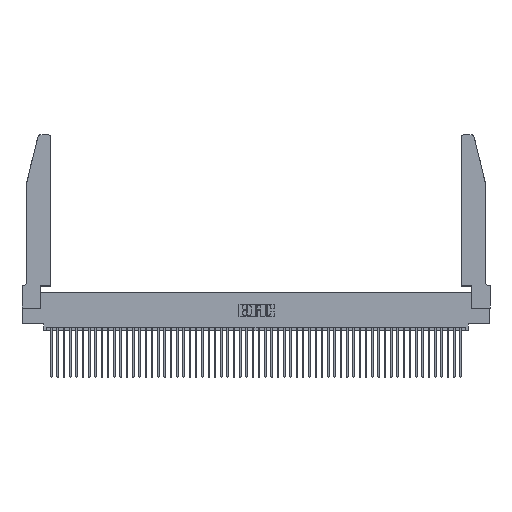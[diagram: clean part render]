
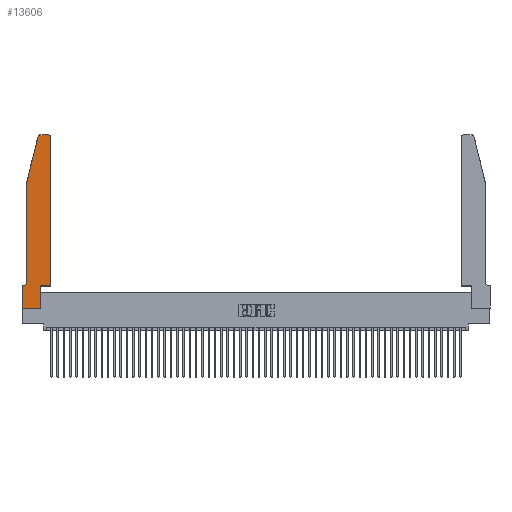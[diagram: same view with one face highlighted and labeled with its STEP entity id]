
A CAD part, top view. The second image highlights one B-rep face of the part: STEP entity #13606.
In plain terms, the highlighted planar face has unit normal (0, 0, 1).
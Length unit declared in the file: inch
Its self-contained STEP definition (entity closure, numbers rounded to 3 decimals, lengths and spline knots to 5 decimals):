
#648 = VERTEX_POINT ( 'NONE', #53403 ) ;
#2303 = EDGE_CURVE ( 'NONE', #8996, #44740, #25401, .T. ) ;
#3065 = ORIENTED_EDGE ( 'NONE', *, *, #2303, .T. ) ;
#3672 = CARTESIAN_POINT ( 'NONE',  ( 0.4505, 0.35, 0.37 ) ) ;
#4632 = AXIS2_PLACEMENT_3D ( 'NONE', #6742, #19001, #35114 ) ;
#5194 = CARTESIAN_POINT ( 'NONE',  ( 0.2865, 0., 0.37 ) ) ;
#5796 = LINE ( 'NONE', #16318, #37480 ) ;
#5951 = CARTESIAN_POINT ( 'NONE',  ( 0., 0., 0.37 ) ) ;
#6228 = CARTESIAN_POINT ( 'NONE',  ( 0.0055, 0.42, 0.37 ) ) ;
#6640 = AXIS2_PLACEMENT_3D ( 'NONE', #6228, #18672, #35143 ) ;
#6742 = CARTESIAN_POINT ( 'NONE',  ( 0.4205, 2.72, 0.37 ) ) ;
#7563 = EDGE_CURVE ( 'NONE', #29577, #43509, #40309, .T. ) ;
#8777 = VECTOR ( 'NONE', #47418, 39.37008 ) ;
#8996 = VERTEX_POINT ( 'NONE', #10641 ) ;
#9211 = DIRECTION ( 'NONE',  ( 0., 1., 0. ) ) ;
#9714 = DIRECTION ( 'NONE',  ( -0.239, -0.971, 0. ) ) ;
#9762 = EDGE_CURVE ( 'NONE', #44667, #41409, #36049, .T. ) ;
#10292 = LINE ( 'NONE', #13333, #30944 ) ;
#10329 = DIRECTION ( 'NONE',  ( -1., 0., 0. ) ) ;
#10641 = CARTESIAN_POINT ( 'NONE',  ( 0.25487, 2.72718, 0.37 ) ) ;
#10679 = EDGE_CURVE ( 'NONE', #43509, #648, #10292, .T. ) ;
#11545 = VERTEX_POINT ( 'NONE', #17422 ) ;
#12199 = ORIENTED_EDGE ( 'NONE', *, *, #41838, .T. ) ;
#12677 = CIRCLE ( 'NONE', #42104, 0.03 ) ;
#13333 = CARTESIAN_POINT ( 'NONE',  ( 0.2605, 2.75, 0.37 ) ) ;
#13467 = ORIENTED_EDGE ( 'NONE', *, *, #7563, .T. ) ;
#13606 = ADVANCED_FACE ( 'NONE', ( #36514 ), #26960, .T. ) ;
#13779 = CARTESIAN_POINT ( 'NONE',  ( 0.4505, 0.35, 0.37 ) ) ;
#13926 = CARTESIAN_POINT ( 'NONE',  ( 0.2865, 0.35, 0.37 ) ) ;
#13992 = VERTEX_POINT ( 'NONE', #14351 ) ;
#14351 = CARTESIAN_POINT ( 'NONE',  ( 0., 0.35, 0.37 ) ) ;
#16318 = CARTESIAN_POINT ( 'NONE',  ( 0.0755, 2., 0.37 ) ) ;
#17422 = CARTESIAN_POINT ( 'NONE',  ( 0.2865, 0.35, 0.37 ) ) ;
#18121 = DIRECTION ( 'NONE',  ( 0., 0., 1. ) ) ;
#18648 = CARTESIAN_POINT ( 'NONE',  ( 0.4505, 2.72, 0.37 ) ) ;
#18672 = DIRECTION ( 'NONE',  ( 0., 0., -1. ) ) ;
#18873 = LINE ( 'NONE', #51528, #42839 ) ;
#19001 = DIRECTION ( 'NONE',  ( 0., 0., 1. ) ) ;
#19073 = CARTESIAN_POINT ( 'NONE',  ( 0.0755, 2., 0.37 ) ) ;
#19145 = EDGE_LOOP ( 'NONE', ( #34666, #48210, #3065, #25283, #41855, #52865, #50032, #31423, #12199, #38672, #34093, #13467 ) ) ;
#20128 = VECTOR ( 'NONE', #9211, 39.37008 ) ;
#20207 = VECTOR ( 'NONE', #9714, 39.37008 ) ;
#20814 = LINE ( 'NONE', #13926, #20128 ) ;
#22872 = EDGE_CURVE ( 'NONE', #43581, #13992, #18873, .T. ) ;
#24949 = CARTESIAN_POINT ( 'NONE',  ( 0., 0., 0.37 ) ) ;
#25047 = VECTOR ( 'NONE', #47370, 39.37008 ) ;
#25283 = ORIENTED_EDGE ( 'NONE', *, *, #36935, .T. ) ;
#25401 = LINE ( 'NONE', #30651, #20207 ) ;
#26869 = LINE ( 'NONE', #38360, #8777 ) ;
#26960 = PLANE ( 'NONE',  #45649 ) ;
#27677 = DIRECTION ( 'NONE',  ( 0., 1., 0. ) ) ;
#27846 = VERTEX_POINT ( 'NONE', #13779 ) ;
#27872 = DIRECTION ( 'NONE',  ( 1., 0., 0. ) ) ;
#29100 = DIRECTION ( 'NONE',  ( 0., -1., 0. ) ) ;
#29577 = VERTEX_POINT ( 'NONE', #18648 ) ;
#30592 = CARTESIAN_POINT ( 'NONE',  ( 0., 0.35, 0.37 ) ) ;
#30651 = CARTESIAN_POINT ( 'NONE',  ( 0.0755, 2., 0.37 ) ) ;
#30944 = VECTOR ( 'NONE', #50217, 39.37008 ) ;
#31423 = ORIENTED_EDGE ( 'NONE', *, *, #9762, .T. ) ;
#32558 = EDGE_CURVE ( 'NONE', #648, #8996, #12677, .T. ) ;
#34093 = ORIENTED_EDGE ( 'NONE', *, *, #43334, .T. ) ;
#34666 = ORIENTED_EDGE ( 'NONE', *, *, #10679, .T. ) ;
#35114 = DIRECTION ( 'NONE',  ( 1., 0., 0. ) ) ;
#35143 = DIRECTION ( 'NONE',  ( -1., 0., 0. ) ) ;
#35899 = CARTESIAN_POINT ( 'NONE',  ( 0., 0., 0.37 ) ) ;
#36049 = LINE ( 'NONE', #5951, #25047 ) ;
#36514 = FACE_OUTER_BOUND ( 'NONE', #19145, .T. ) ;
#36935 = EDGE_CURVE ( 'NONE', #44740, #43360, #5796, .T. ) ;
#37480 = VECTOR ( 'NONE', #48894, 39.37008 ) ;
#37617 = CARTESIAN_POINT ( 'NONE',  ( 0.0755, 0.42, 0.37 ) ) ;
#38324 = CARTESIAN_POINT ( 'NONE',  ( 0.0055, 0.35, 0.37 ) ) ;
#38360 = CARTESIAN_POINT ( 'NONE',  ( 0.4505, 0.35, 0.37 ) ) ;
#38627 = EDGE_CURVE ( 'NONE', #13992, #44667, #53421, .T. ) ;
#38672 = ORIENTED_EDGE ( 'NONE', *, *, #47986, .T. ) ;
#38924 = DIRECTION ( 'NONE',  ( 1., 0., 0. ) ) ;
#40072 = LINE ( 'NONE', #3672, #42685 ) ;
#40309 = CIRCLE ( 'NONE', #4632, 0.03 ) ;
#40725 = CARTESIAN_POINT ( 'NONE',  ( 0.284, 2.72, 0.37 ) ) ;
#41409 = VERTEX_POINT ( 'NONE', #5194 ) ;
#41838 = EDGE_CURVE ( 'NONE', #41409, #11545, #20814, .T. ) ;
#41855 = ORIENTED_EDGE ( 'NONE', *, *, #47282, .T. ) ;
#42104 = AXIS2_PLACEMENT_3D ( 'NONE', #40725, #44908, #27872 ) ;
#42685 = VECTOR ( 'NONE', #27677, 39.37008 ) ;
#42839 = VECTOR ( 'NONE', #10329, 39.37008 ) ;
#43095 = VECTOR ( 'NONE', #29100, 39.37008 ) ;
#43334 = EDGE_CURVE ( 'NONE', #27846, #29577, #40072, .T. ) ;
#43360 = VERTEX_POINT ( 'NONE', #37617 ) ;
#43509 = VERTEX_POINT ( 'NONE', #50630 ) ;
#43581 = VERTEX_POINT ( 'NONE', #38324 ) ;
#44667 = VERTEX_POINT ( 'NONE', #35899 ) ;
#44740 = VERTEX_POINT ( 'NONE', #19073 ) ;
#44908 = DIRECTION ( 'NONE',  ( 0., 0., 1. ) ) ;
#45649 = AXIS2_PLACEMENT_3D ( 'NONE', #30592, #18121, #38924 ) ;
#47282 = EDGE_CURVE ( 'NONE', #43360, #43581, #50918, .T. ) ;
#47370 = DIRECTION ( 'NONE',  ( 1., 0., 0. ) ) ;
#47418 = DIRECTION ( 'NONE',  ( 1., 0., 0. ) ) ;
#47986 = EDGE_CURVE ( 'NONE', #11545, #27846, #26869, .T. ) ;
#48210 = ORIENTED_EDGE ( 'NONE', *, *, #32558, .T. ) ;
#48894 = DIRECTION ( 'NONE',  ( 0., -1., 0. ) ) ;
#50032 = ORIENTED_EDGE ( 'NONE', *, *, #38627, .T. ) ;
#50217 = DIRECTION ( 'NONE',  ( -1., 0., 0. ) ) ;
#50630 = CARTESIAN_POINT ( 'NONE',  ( 0.4205, 2.75, 0.37 ) ) ;
#50918 = CIRCLE ( 'NONE', #6640, 0.07 ) ;
#51528 = CARTESIAN_POINT ( 'NONE',  ( 0.0755, 0.35, 0.37 ) ) ;
#52865 = ORIENTED_EDGE ( 'NONE', *, *, #22872, .T. ) ;
#53403 = CARTESIAN_POINT ( 'NONE',  ( 0.284, 2.75, 0.37 ) ) ;
#53421 = LINE ( 'NONE', #24949, #43095 ) ;
